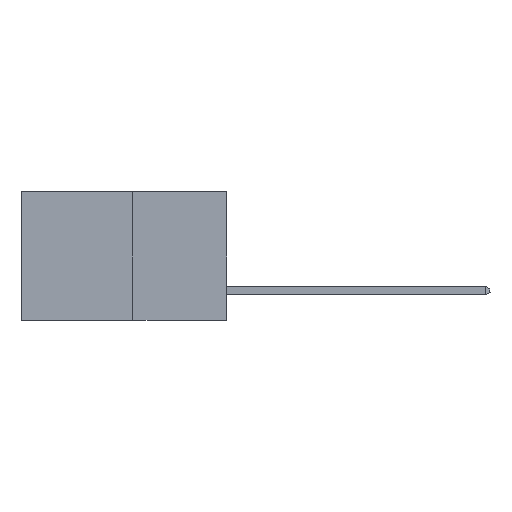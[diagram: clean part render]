
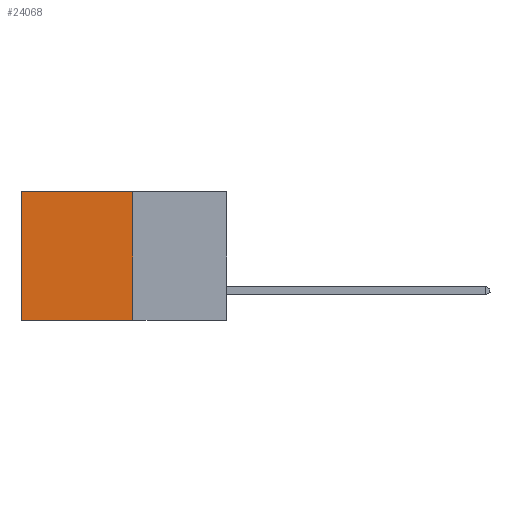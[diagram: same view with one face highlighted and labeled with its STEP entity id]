
A CAD part, left-side view. The second image highlights one B-rep face of the part: STEP entity #24068.
In plain terms, the highlighted planar face has unit normal (-1, 0, 0).
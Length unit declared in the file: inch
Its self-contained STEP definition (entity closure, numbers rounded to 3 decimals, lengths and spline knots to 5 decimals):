
#1115 = AXIS2_PLACEMENT_3D ( 'NONE', #14315, #31861, #16822 ) ;
#3388 = LINE ( 'NONE', #21383, #9412 ) ;
#4462 = VECTOR ( 'NONE', #18797, 39.37008 ) ;
#4624 = ORIENTED_EDGE ( 'NONE', *, *, #22312, .T. ) ;
#5270 = EDGE_CURVE ( 'NONE', #12317, #14267, #17926, .T. ) ;
#6295 = DIRECTION ( 'NONE',  ( 0., 1., 0. ) ) ;
#6545 = FACE_OUTER_BOUND ( 'NONE', #27242, .T. ) ;
#7501 = CARTESIAN_POINT ( 'NONE',  ( 0.277, 0.59, -0.37 ) ) ;
#7986 = CARTESIAN_POINT ( 'NONE',  ( 0.277, 0.59, 0. ) ) ;
#8708 = VERTEX_POINT ( 'NONE', #25586 ) ;
#9412 = VECTOR ( 'NONE', #6295, 39.37008 ) ;
#10074 = DIRECTION ( 'NONE',  ( 0., 0., -1. ) ) ;
#12317 = VERTEX_POINT ( 'NONE', #29084 ) ;
#12504 = VECTOR ( 'NONE', #24749, 39.37008 ) ;
#14267 = VERTEX_POINT ( 'NONE', #16798 ) ;
#14315 = CARTESIAN_POINT ( 'NONE',  ( 0.277, 0.27, -0.37 ) ) ;
#16798 = CARTESIAN_POINT ( 'NONE',  ( 0.277, 0.27, -0.37 ) ) ;
#16822 = DIRECTION ( 'NONE',  ( 0., 0., -1. ) ) ;
#17772 = EDGE_CURVE ( 'NONE', #12317, #24704, #3388, .T. ) ;
#17926 = LINE ( 'NONE', #24182, #4462 ) ;
#18797 = DIRECTION ( 'NONE',  ( 0., 0., -1. ) ) ;
#19225 = PLANE ( 'NONE',  #1115 ) ;
#19663 = LINE ( 'NONE', #7501, #32229 ) ;
#21383 = CARTESIAN_POINT ( 'NONE',  ( 0.277, 0.27, 0. ) ) ;
#22188 = ORIENTED_EDGE ( 'NONE', *, *, #24485, .F. ) ;
#22207 = CARTESIAN_POINT ( 'NONE',  ( 0.277, 0.27, -0.37 ) ) ;
#22312 = EDGE_CURVE ( 'NONE', #24704, #8708, #19663, .T. ) ;
#24068 = ADVANCED_FACE ( 'NONE', ( #6545 ), #19225, .F. ) ;
#24182 = CARTESIAN_POINT ( 'NONE',  ( 0.277, 0.27, -0.37 ) ) ;
#24485 = EDGE_CURVE ( 'NONE', #14267, #8708, #32517, .T. ) ;
#24576 = ORIENTED_EDGE ( 'NONE', *, *, #5270, .F. ) ;
#24704 = VERTEX_POINT ( 'NONE', #7986 ) ;
#24749 = DIRECTION ( 'NONE',  ( 0., 1., 0. ) ) ;
#25586 = CARTESIAN_POINT ( 'NONE',  ( 0.277, 0.59, -0.37 ) ) ;
#27242 = EDGE_LOOP ( 'NONE', ( #4624, #22188, #24576, #27723 ) ) ;
#27723 = ORIENTED_EDGE ( 'NONE', *, *, #17772, .T. ) ;
#29084 = CARTESIAN_POINT ( 'NONE',  ( 0.277, 0.27, 0. ) ) ;
#31861 = DIRECTION ( 'NONE',  ( 1., 0., 0. ) ) ;
#32229 = VECTOR ( 'NONE', #10074, 39.37008 ) ;
#32517 = LINE ( 'NONE', #22207, #12504 ) ;
